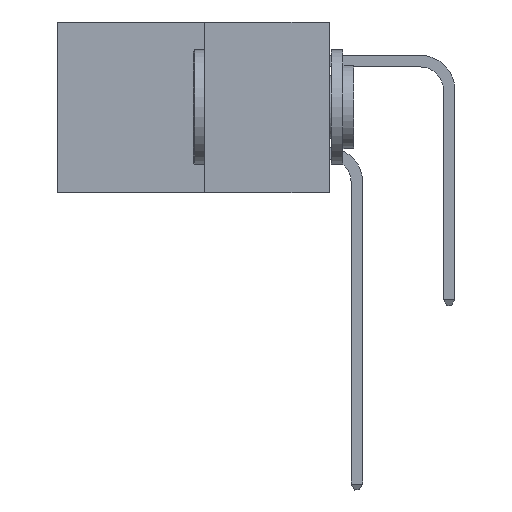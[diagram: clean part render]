
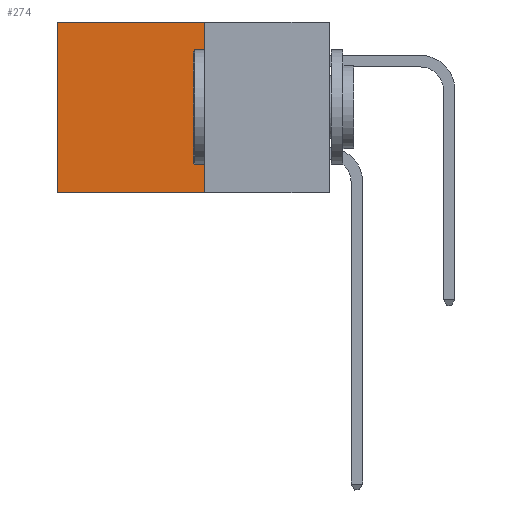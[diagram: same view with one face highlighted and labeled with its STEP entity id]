
A CAD part, left-side view. The second image highlights one B-rep face of the part: STEP entity #274.
In plain terms, the highlighted planar face has unit normal (-1, 0, 0).
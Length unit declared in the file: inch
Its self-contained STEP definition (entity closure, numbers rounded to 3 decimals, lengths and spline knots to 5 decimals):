
#274 = ADVANCED_FACE ( 'NONE', ( #16988 ), #8141, .F. ) ;
#2344 = VERTEX_POINT ( 'NONE', #4364 ) ;
#2883 = VECTOR ( 'NONE', #11571, 39.37008 ) ;
#3080 = EDGE_CURVE ( 'NONE', #3478, #21758, #7457, .T. ) ;
#3478 = VERTEX_POINT ( 'NONE', #7468 ) ;
#4364 = CARTESIAN_POINT ( 'NONE',  ( 0.277, 0.59, 0. ) ) ;
#4692 = VECTOR ( 'NONE', #12814, 39.37008 ) ;
#4755 = DIRECTION ( 'NONE',  ( 1., 0., 0. ) ) ;
#5324 = ORIENTED_EDGE ( 'NONE', *, *, #17729, .T. ) ;
#5426 = EDGE_CURVE ( 'NONE', #21758, #23127, #22663, .T. ) ;
#6063 = ORIENTED_EDGE ( 'NONE', *, *, #5426, .F. ) ;
#7426 = LINE ( 'NONE', #14701, #17300 ) ;
#7457 = LINE ( 'NONE', #13884, #12422 ) ;
#7468 = CARTESIAN_POINT ( 'NONE',  ( 0.277, 0.27, 0. ) ) ;
#8141 = PLANE ( 'NONE',  #20564 ) ;
#9471 = CARTESIAN_POINT ( 'NONE',  ( 0.277, 0.27, -0.37 ) ) ;
#10153 = DIRECTION ( 'NONE',  ( 0., 0., -1. ) ) ;
#10866 = LINE ( 'NONE', #18285, #4692 ) ;
#11107 = ORIENTED_EDGE ( 'NONE', *, *, #3080, .F. ) ;
#11293 = CARTESIAN_POINT ( 'NONE',  ( 0.277, 0.59, -0.37 ) ) ;
#11571 = DIRECTION ( 'NONE',  ( 0., 1., 0. ) ) ;
#11699 = CARTESIAN_POINT ( 'NONE',  ( 0.277, 0.27, -0.37 ) ) ;
#12422 = VECTOR ( 'NONE', #12647, 39.37008 ) ;
#12647 = DIRECTION ( 'NONE',  ( 0., 0., -1. ) ) ;
#12814 = DIRECTION ( 'NONE',  ( 0., 0., -1. ) ) ;
#13685 = ORIENTED_EDGE ( 'NONE', *, *, #23748, .T. ) ;
#13884 = CARTESIAN_POINT ( 'NONE',  ( 0.277, 0.27, -0.37 ) ) ;
#14701 = CARTESIAN_POINT ( 'NONE',  ( 0.277, 0.27, 0. ) ) ;
#16352 = EDGE_LOOP ( 'NONE', ( #13685, #6063, #11107, #5324 ) ) ;
#16525 = CARTESIAN_POINT ( 'NONE',  ( 0.277, 0.27, -0.37 ) ) ;
#16988 = FACE_OUTER_BOUND ( 'NONE', #16352, .T. ) ;
#17300 = VECTOR ( 'NONE', #18318, 39.37008 ) ;
#17729 = EDGE_CURVE ( 'NONE', #3478, #2344, #7426, .T. ) ;
#18285 = CARTESIAN_POINT ( 'NONE',  ( 0.277, 0.59, -0.37 ) ) ;
#18318 = DIRECTION ( 'NONE',  ( 0., 1., 0. ) ) ;
#20564 = AXIS2_PLACEMENT_3D ( 'NONE', #16525, #4755, #10153 ) ;
#21758 = VERTEX_POINT ( 'NONE', #9471 ) ;
#22663 = LINE ( 'NONE', #11699, #2883 ) ;
#23127 = VERTEX_POINT ( 'NONE', #11293 ) ;
#23748 = EDGE_CURVE ( 'NONE', #2344, #23127, #10866, .T. ) ;
